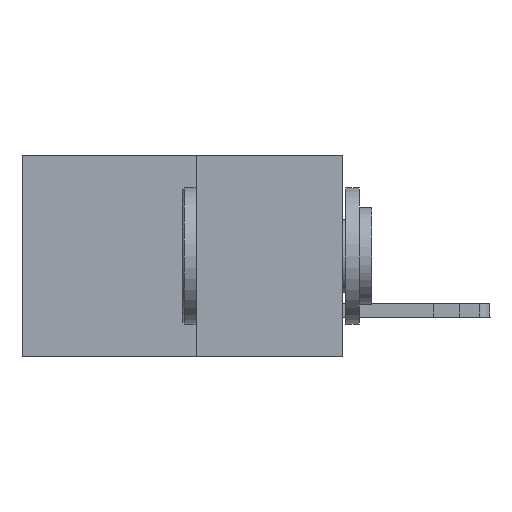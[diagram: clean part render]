
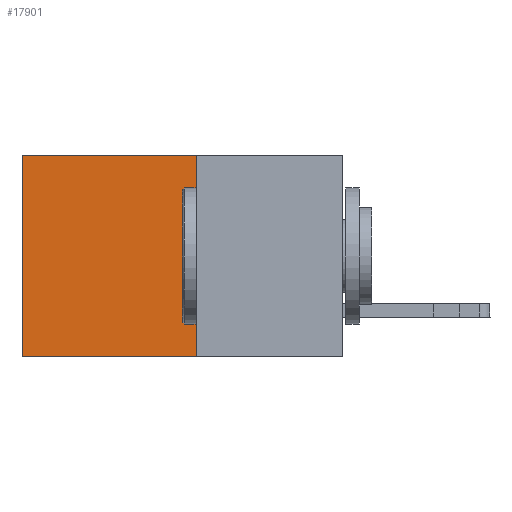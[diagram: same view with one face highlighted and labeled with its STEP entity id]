
A CAD part, left-side view. The second image highlights one B-rep face of the part: STEP entity #17901.
In plain terms, the highlighted planar face has unit normal (-1, 0, 0).
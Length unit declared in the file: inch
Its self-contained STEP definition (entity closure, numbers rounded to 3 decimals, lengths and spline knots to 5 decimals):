
#113 = ORIENTED_EDGE ( 'NONE', *, *, #1056, .F. ) ;
#1056 = EDGE_CURVE ( 'NONE', #21542, #22474, #6442, .T. ) ;
#1367 = VECTOR ( 'NONE', #24314, 39.37008 ) ;
#1579 = DIRECTION ( 'NONE',  ( 0., 0., -1. ) ) ;
#1776 = LINE ( 'NONE', #21195, #15857 ) ;
#2111 = CARTESIAN_POINT ( 'NONE',  ( 0.277, 0.27, -0.37 ) ) ;
#2873 = PLANE ( 'NONE',  #25166 ) ;
#4820 = FACE_OUTER_BOUND ( 'NONE', #19974, .T. ) ;
#5002 = EDGE_CURVE ( 'NONE', #22474, #17806, #1776, .T. ) ;
#6361 = ORIENTED_EDGE ( 'NONE', *, *, #24022, .T. ) ;
#6442 = LINE ( 'NONE', #10767, #21790 ) ;
#6596 = EDGE_CURVE ( 'NONE', #17667, #17806, #14151, .T. ) ;
#7492 = ORIENTED_EDGE ( 'NONE', *, *, #5002, .F. ) ;
#7829 = ORIENTED_EDGE ( 'NONE', *, *, #6596, .T. ) ;
#8679 = DIRECTION ( 'NONE',  ( 0., 0., -1. ) ) ;
#9287 = DIRECTION ( 'NONE',  ( 1., 0., 0. ) ) ;
#9359 = LINE ( 'NONE', #17874, #1367 ) ;
#10712 = DIRECTION ( 'NONE',  ( 0., 1., 0. ) ) ;
#10767 = CARTESIAN_POINT ( 'NONE',  ( 0.277, 0.27, -0.37 ) ) ;
#11397 = CARTESIAN_POINT ( 'NONE',  ( 0.277, 0.27, -0.37 ) ) ;
#14151 = LINE ( 'NONE', #22662, #22571 ) ;
#15857 = VECTOR ( 'NONE', #10712, 39.37008 ) ;
#17667 = VERTEX_POINT ( 'NONE', #25650 ) ;
#17802 = DIRECTION ( 'NONE',  ( 0., 0., -1. ) ) ;
#17806 = VERTEX_POINT ( 'NONE', #24098 ) ;
#17874 = CARTESIAN_POINT ( 'NONE',  ( 0.277, 0.27, 0. ) ) ;
#17901 = ADVANCED_FACE ( 'NONE', ( #4820 ), #2873, .F. ) ;
#19974 = EDGE_LOOP ( 'NONE', ( #7829, #7492, #113, #6361 ) ) ;
#21195 = CARTESIAN_POINT ( 'NONE',  ( 0.277, 0.27, -0.37 ) ) ;
#21542 = VERTEX_POINT ( 'NONE', #27009 ) ;
#21790 = VECTOR ( 'NONE', #8679, 39.37008 ) ;
#22474 = VERTEX_POINT ( 'NONE', #2111 ) ;
#22571 = VECTOR ( 'NONE', #1579, 39.37008 ) ;
#22662 = CARTESIAN_POINT ( 'NONE',  ( 0.277, 0.59, -0.37 ) ) ;
#24022 = EDGE_CURVE ( 'NONE', #21542, #17667, #9359, .T. ) ;
#24098 = CARTESIAN_POINT ( 'NONE',  ( 0.277, 0.59, -0.37 ) ) ;
#24314 = DIRECTION ( 'NONE',  ( 0., 1., 0. ) ) ;
#25166 = AXIS2_PLACEMENT_3D ( 'NONE', #11397, #9287, #17802 ) ;
#25650 = CARTESIAN_POINT ( 'NONE',  ( 0.277, 0.59, 0. ) ) ;
#27009 = CARTESIAN_POINT ( 'NONE',  ( 0.277, 0.27, 0. ) ) ;
